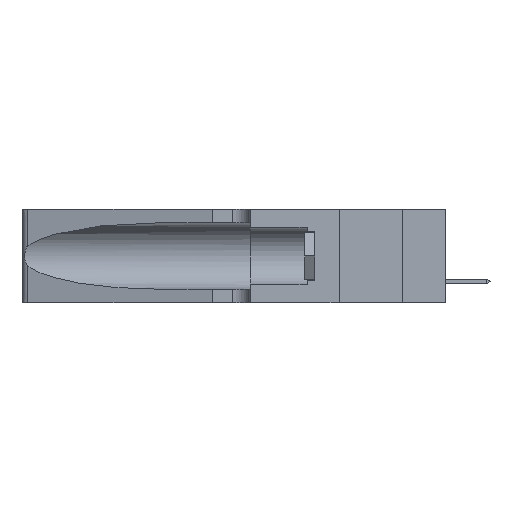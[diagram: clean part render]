
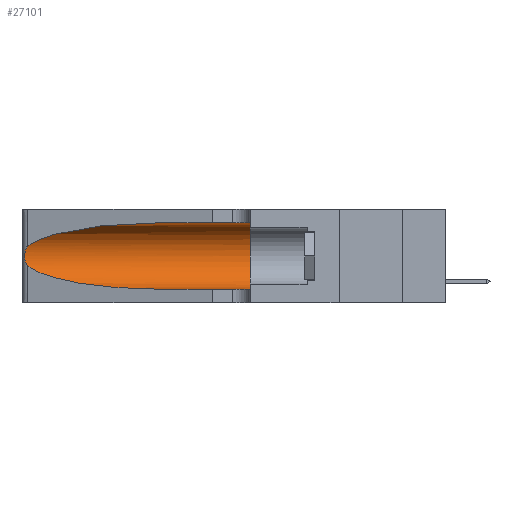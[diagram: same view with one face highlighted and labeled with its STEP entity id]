
A CAD part, left-side view. The second image highlights one B-rep face of the part: STEP entity #27101.
In plain terms, the highlighted cylindrical face has radius 3.308 mm (diameter 6.617 mm), a partial arc.
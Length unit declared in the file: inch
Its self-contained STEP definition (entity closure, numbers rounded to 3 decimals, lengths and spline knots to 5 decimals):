
#122 = CARTESIAN_POINT ( 'NONE',  ( 0.25639, 1.23186, 0.15144 ) ) ;
#913 = EDGE_CURVE ( 'NONE', #25399, #32586, #19111, .T. ) ;
#1955 = CARTESIAN_POINT ( 'NONE',  ( 0.1305, 0.72297, 0.05475 ) ) ;
#2506 = EDGE_CURVE ( 'NONE', #27490, #4505, #41554, .T. ) ;
#3183 = CARTESIAN_POINT ( 'NONE',  ( 0.26075, 1.23896, 0.19203 ) ) ;
#3458 = CARTESIAN_POINT ( 'NONE',  ( 0.25555, 1.22994, 0.2215 ) ) ;
#4505 = VERTEX_POINT ( 'NONE', #1955 ) ;
#5114 = ORIENTED_EDGE ( 'NONE', *, *, #38140, .F. ) ;
#6170 = DIRECTION ( 'NONE',  ( 0., -1., 0. ) ) ;
#6532 = CARTESIAN_POINT ( 'NONE',  ( 0.26017, 1.23833, 0.17102 ) ) ;
#6669 = CARTESIAN_POINT ( 'NONE',  ( 0.25487, 1.22718, 0.14631 ) ) ;
#7058 = CARTESIAN_POINT ( 'NONE',  ( 0.1305, 0.35, 0.31525 ) ) ;
#7070 = FACE_OUTER_BOUND ( 'NONE', #33332, .T. ) ;
#7584 = ORIENTED_EDGE ( 'NONE', *, *, #2506, .T. ) ;
#8456 = CARTESIAN_POINT ( 'NONE',  ( 0.1305, 0.72297, 0.31525 ) ) ;
#10043 = CARTESIAN_POINT ( 'NONE',  ( 0.26018, 1.23835, 0.19895 ) ) ;
#10096 = VERTEX_POINT ( 'NONE', #28734 ) ;
#11152 = ORIENTED_EDGE ( 'NONE', *, *, #29459, .T. ) ;
#11194 = DIRECTION ( 'NONE',  ( 0., -1., 0. ) ) ;
#12521 = VERTEX_POINT ( 'NONE', #20946 ) ;
#12804 = VECTOR ( 'NONE', #29874, 39.37008 ) ;
#13450 = CIRCLE ( 'NONE', #33755, 0.13025 ) ;
#13573 = CARTESIAN_POINT ( 'NONE',  ( 0.25487, 1.22718, 0.14631 ) ) ;
#15590 = B_SPLINE_CURVE_WITH_KNOTS ( 'NONE', 3,
 ( #36630, #3458, #36496, #16675, #39845, #10043, #3183, #26619, #6532, #20023, #23385, #122, #26753, #6669 ),
 .UNSPECIFIED., .F., .F.,
 ( 4, 2, 2, 2, 2, 2, 4 ),
 ( 0., 0.00027, 0.00053, 0.00107, 0.0016, 0.00187, 0.00214 ),
 .UNSPECIFIED. ) ;
#16675 = CARTESIAN_POINT ( 'NONE',  ( 0.25787, 1.23484, 0.2124 ) ) ;
#17166 = ORIENTED_EDGE ( 'NONE', *, *, #913, .F. ) ;
#19111 = LINE ( 'NONE', #32351, #12804 ) ;
#20023 = CARTESIAN_POINT ( 'NONE',  ( 0.25856, 1.23593, 0.16098 ) ) ;
#20946 = CARTESIAN_POINT ( 'NONE',  ( 0.25487, 1.22718, 0.22369 ) ) ;
#22135 = EDGE_CURVE ( 'NONE', #12521, #27490, #15590, .T. ) ;
#22748 = AXIS2_PLACEMENT_3D ( 'NONE', #28046, #11194, #24688 ) ;
#22793 = CARTESIAN_POINT ( 'NONE',  ( 0.18966, 0.96281, 0.05475 ) ) ;
#23385 = CARTESIAN_POINT ( 'NONE',  ( 0.25789, 1.23486, 0.15765 ) ) ;
#24688 = DIRECTION ( 'NONE',  ( 0., 0., -1. ) ) ;
#24720 =( BOUNDED_CURVE ( )  B_SPLINE_CURVE ( 3, ( #8456, #25456, #31704, #42211 ),
 .UNSPECIFIED., .F., .F. ) 
 B_SPLINE_CURVE_WITH_KNOTS ( ( 4, 4 ),
 ( 1.5708, 2.84003 ),
 .UNSPECIFIED. ) 
 CURVE ( )  GEOMETRIC_REPRESENTATION_ITEM ( )  RATIONAL_B_SPLINE_CURVE ( ( 1., 0.87, 0.87, 1. ) ) 
 REPRESENTATION_ITEM ( '' )  );
#24817 = ORIENTED_EDGE ( 'NONE', *, *, #27325, .T. ) ;
#25399 = VERTEX_POINT ( 'NONE', #26533 ) ;
#25456 = CARTESIAN_POINT ( 'NONE',  ( 0.18966, 0.96281, 0.31525 ) ) ;
#26104 = DIRECTION ( 'NONE',  ( 0., 0., 1. ) ) ;
#26533 = CARTESIAN_POINT ( 'NONE',  ( 0.1305, 0.72297, 0.31525 ) ) ;
#26619 = CARTESIAN_POINT ( 'NONE',  ( 0.26075, 1.23896, 0.178 ) ) ;
#26753 = CARTESIAN_POINT ( 'NONE',  ( 0.25555, 1.22993, 0.14849 ) ) ;
#26976 = CARTESIAN_POINT ( 'NONE',  ( 0.25487, 1.22718, 0.14631 ) ) ;
#27101 = ADVANCED_FACE ( 'NONE', ( #7070 ), #28561, .F. ) ;
#27325 = EDGE_CURVE ( 'NONE', #4505, #10096, #28023, .T. ) ;
#27490 = VERTEX_POINT ( 'NONE', #26976 ) ;
#28023 = LINE ( 'NONE', #42741, #42117 ) ;
#28046 = CARTESIAN_POINT ( 'NONE',  ( 0.1305, 1.61858, 0.185 ) ) ;
#28561 = CYLINDRICAL_SURFACE ( 'NONE', #22748, 0.13025 ) ;
#28734 = CARTESIAN_POINT ( 'NONE',  ( 0.1305, 0.35, 0.05475 ) ) ;
#29459 = EDGE_CURVE ( 'NONE', #25399, #12521, #24720, .T. ) ;
#29874 = DIRECTION ( 'NONE',  ( 0., -1., 0. ) ) ;
#31704 = CARTESIAN_POINT ( 'NONE',  ( 0.2373, 1.15595, 0.28018 ) ) ;
#32351 = CARTESIAN_POINT ( 'NONE',  ( 0.1305, 1.61858, 0.31525 ) ) ;
#32586 = VERTEX_POINT ( 'NONE', #7058 ) ;
#33332 = EDGE_LOOP ( 'NONE', ( #11152, #33596, #7584, #24817, #5114, #17166 ) ) ;
#33596 = ORIENTED_EDGE ( 'NONE', *, *, #22135, .T. ) ;
#33755 = AXIS2_PLACEMENT_3D ( 'NONE', #36265, #42713, #26104 ) ;
#34443 = CARTESIAN_POINT ( 'NONE',  ( 0.2373, 1.15595, 0.08982 ) ) ;
#36265 = CARTESIAN_POINT ( 'NONE',  ( 0.1305, 0.35, 0.185 ) ) ;
#36496 = CARTESIAN_POINT ( 'NONE',  ( 0.25639, 1.23184, 0.21858 ) ) ;
#36630 = CARTESIAN_POINT ( 'NONE',  ( 0.25487, 1.22718, 0.22369 ) ) ;
#38140 = EDGE_CURVE ( 'NONE', #32586, #10096, #13450, .T. ) ;
#39845 = CARTESIAN_POINT ( 'NONE',  ( 0.25854, 1.2359, 0.20912 ) ) ;
#41554 =( BOUNDED_CURVE ( )  B_SPLINE_CURVE ( 3, ( #13573, #34443, #22793, #42895 ),
 .UNSPECIFIED., .F., .T. ) 
 B_SPLINE_CURVE_WITH_KNOTS ( ( 4, 4 ),
 ( 3.44316, 4.71239 ),
 .UNSPECIFIED. ) 
 CURVE ( )  GEOMETRIC_REPRESENTATION_ITEM ( )  RATIONAL_B_SPLINE_CURVE ( ( 1., 0.87, 0.87, 1. ) ) 
 REPRESENTATION_ITEM ( '' )  );
#42117 = VECTOR ( 'NONE', #6170, 39.37008 ) ;
#42211 = CARTESIAN_POINT ( 'NONE',  ( 0.25487, 1.22718, 0.22369 ) ) ;
#42713 = DIRECTION ( 'NONE',  ( 0., 1., 0. ) ) ;
#42741 = CARTESIAN_POINT ( 'NONE',  ( 0.1305, 1.61858, 0.05475 ) ) ;
#42895 = CARTESIAN_POINT ( 'NONE',  ( 0.1305, 0.72297, 0.05475 ) ) ;
